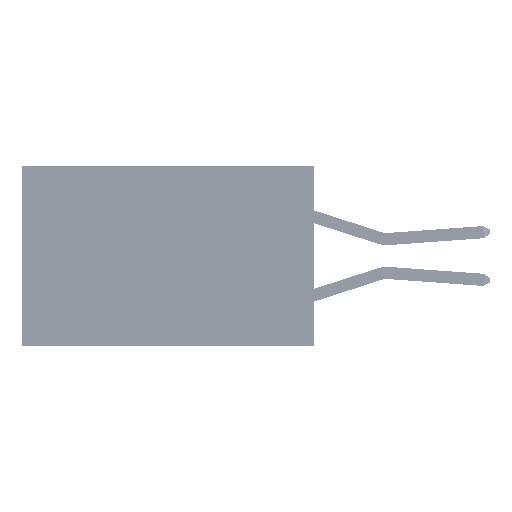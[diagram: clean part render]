
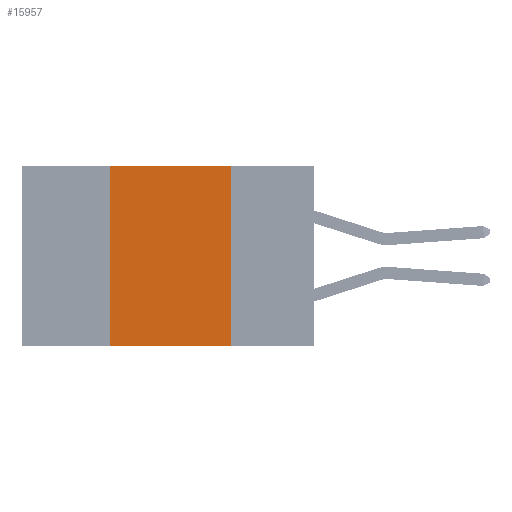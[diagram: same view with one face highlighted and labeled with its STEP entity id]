
A CAD part, left-side view. The second image highlights one B-rep face of the part: STEP entity #15957.
In plain terms, the highlighted planar face has unit normal (-1, 0, 0).
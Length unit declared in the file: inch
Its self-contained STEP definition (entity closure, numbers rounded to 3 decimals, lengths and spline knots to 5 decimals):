
#1871 = DIRECTION ( 'NONE',  ( 0., -1., 0. ) ) ;
#5061 = ORIENTED_EDGE ( 'NONE', *, *, #45926, .F. ) ;
#5125 = ORIENTED_EDGE ( 'NONE', *, *, #5711, .F. ) ;
#5711 = EDGE_CURVE ( 'NONE', #28065, #28554, #5788, .T. ) ;
#5788 = LINE ( 'NONE', #32631, #26228 ) ;
#7041 = DIRECTION ( 'NONE',  ( 1., 0., 0. ) ) ;
#9338 = VECTOR ( 'NONE', #1871, 39.37008 ) ;
#10502 = CARTESIAN_POINT ( 'NONE',  ( 0., 0.6, 0. ) ) ;
#10846 = EDGE_LOOP ( 'NONE', ( #5125, #50775, #5061, #46314 ) ) ;
#13902 = CARTESIAN_POINT ( 'NONE',  ( 0., 0.6, 0. ) ) ;
#14267 = PLANE ( 'NONE',  #50631 ) ;
#15598 = CARTESIAN_POINT ( 'NONE',  ( 0., 0.42, 0. ) ) ;
#15957 = ADVANCED_FACE ( 'NONE', ( #17939 ), #14267, .F. ) ;
#16531 = CARTESIAN_POINT ( 'NONE',  ( 0., 0.6, -0.37 ) ) ;
#17242 = VECTOR ( 'NONE', #20002, 39.37008 ) ;
#17939 = FACE_OUTER_BOUND ( 'NONE', #10846, .T. ) ;
#19046 = LINE ( 'NONE', #15598, #43912 ) ;
#19598 = DIRECTION ( 'NONE',  ( 0., 0., 1. ) ) ;
#20002 = DIRECTION ( 'NONE',  ( 0., -1., 0. ) ) ;
#26228 = VECTOR ( 'NONE', #40619, 39.37008 ) ;
#27369 = CARTESIAN_POINT ( 'NONE',  ( 0., 0.42, 0. ) ) ;
#27926 = LINE ( 'NONE', #13902, #9338 ) ;
#28065 = VERTEX_POINT ( 'NONE', #32231 ) ;
#28554 = VERTEX_POINT ( 'NONE', #42948 ) ;
#32231 = CARTESIAN_POINT ( 'NONE',  ( 0., 0.17, 0. ) ) ;
#32631 = CARTESIAN_POINT ( 'NONE',  ( 0., 0.17, 0. ) ) ;
#35773 = VERTEX_POINT ( 'NONE', #27369 ) ;
#36292 = CARTESIAN_POINT ( 'NONE',  ( 0., 0.42, -0.37 ) ) ;
#40619 = DIRECTION ( 'NONE',  ( 0., 0., -1. ) ) ;
#41202 = EDGE_CURVE ( 'NONE', #35773, #28065, #27926, .T. ) ;
#41650 = VERTEX_POINT ( 'NONE', #36292 ) ;
#42402 = DIRECTION ( 'NONE',  ( 0., 0., -1. ) ) ;
#42948 = CARTESIAN_POINT ( 'NONE',  ( 0., 0.17, -0.37 ) ) ;
#43912 = VECTOR ( 'NONE', #19598, 39.37008 ) ;
#45358 = EDGE_CURVE ( 'NONE', #41650, #28554, #45841, .T. ) ;
#45841 = LINE ( 'NONE', #16531, #17242 ) ;
#45926 = EDGE_CURVE ( 'NONE', #41650, #35773, #19046, .T. ) ;
#46314 = ORIENTED_EDGE ( 'NONE', *, *, #45358, .T. ) ;
#50631 = AXIS2_PLACEMENT_3D ( 'NONE', #10502, #7041, #42402 ) ;
#50775 = ORIENTED_EDGE ( 'NONE', *, *, #41202, .F. ) ;
